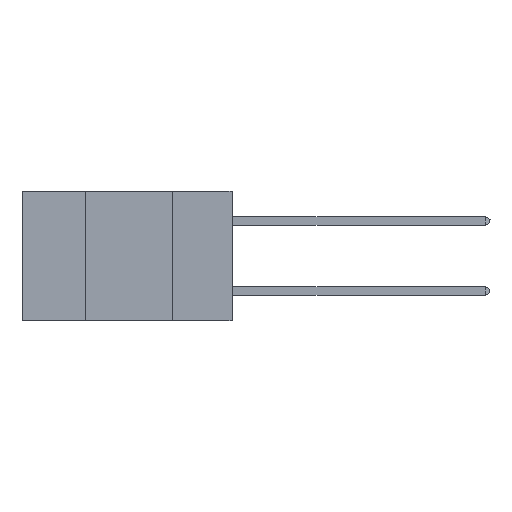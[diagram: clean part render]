
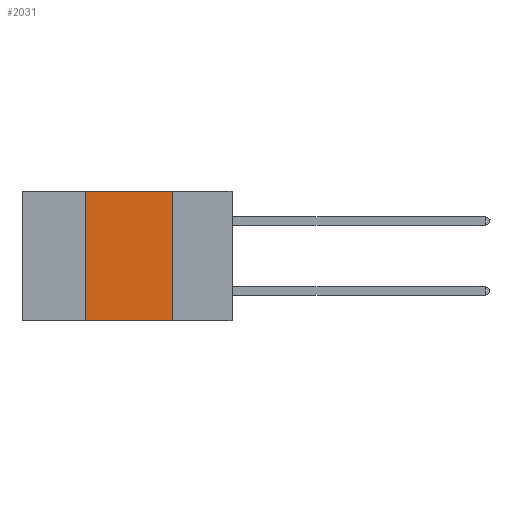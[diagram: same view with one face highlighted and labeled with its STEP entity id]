
A CAD part, left-side view. The second image highlights one B-rep face of the part: STEP entity #2031.
In plain terms, the highlighted planar face has unit normal (-1, 0, 0).
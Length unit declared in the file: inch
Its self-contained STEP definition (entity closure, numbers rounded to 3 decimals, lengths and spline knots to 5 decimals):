
#531 = DIRECTION ( 'NONE',  ( 0., 0., 1. ) ) ;
#580 = EDGE_CURVE ( 'NONE', #26823, #16177, #17739, .T. ) ;
#1506 = DIRECTION ( 'NONE',  ( 0., -1., 0. ) ) ;
#1813 = ORIENTED_EDGE ( 'NONE', *, *, #7496, .F. ) ;
#2031 = ADVANCED_FACE ( 'NONE', ( #20813 ), #12401, .F. ) ;
#2647 = ORIENTED_EDGE ( 'NONE', *, *, #580, .T. ) ;
#3221 = CARTESIAN_POINT ( 'NONE',  ( 0., 0.42, -0.37 ) ) ;
#3333 = CARTESIAN_POINT ( 'NONE',  ( 0., 0.6, 0. ) ) ;
#4228 = CARTESIAN_POINT ( 'NONE',  ( 0., 0.17, 0. ) ) ;
#5326 = VERTEX_POINT ( 'NONE', #15257 ) ;
#6355 = LINE ( 'NONE', #4228, #32613 ) ;
#7496 = EDGE_CURVE ( 'NONE', #26823, #5326, #14928, .T. ) ;
#8200 = CARTESIAN_POINT ( 'NONE',  ( 0., 0.42, 0. ) ) ;
#9907 = VECTOR ( 'NONE', #31317, 39.37008 ) ;
#10989 = CARTESIAN_POINT ( 'NONE',  ( 0., 0.17, -0.37 ) ) ;
#11143 = EDGE_CURVE ( 'NONE', #19741, #16177, #6355, .T. ) ;
#12401 = PLANE ( 'NONE',  #16261 ) ;
#13362 = EDGE_LOOP ( 'NONE', ( #13890, #20681, #1813, #2647 ) ) ;
#13890 = ORIENTED_EDGE ( 'NONE', *, *, #11143, .F. ) ;
#14087 = VECTOR ( 'NONE', #531, 39.37008 ) ;
#14613 = DIRECTION ( 'NONE',  ( 0., 0., -1. ) ) ;
#14928 = LINE ( 'NONE', #8200, #14087 ) ;
#15153 = DIRECTION ( 'NONE',  ( 0., 0., -1. ) ) ;
#15257 = CARTESIAN_POINT ( 'NONE',  ( 0., 0.42, 0. ) ) ;
#16177 = VERTEX_POINT ( 'NONE', #10989 ) ;
#16261 = AXIS2_PLACEMENT_3D ( 'NONE', #27712, #30237, #15153 ) ;
#16936 = VECTOR ( 'NONE', #1506, 39.37008 ) ;
#16974 = CARTESIAN_POINT ( 'NONE',  ( 0., 0.6, -0.37 ) ) ;
#17577 = LINE ( 'NONE', #3333, #9907 ) ;
#17739 = LINE ( 'NONE', #16974, #16936 ) ;
#19741 = VERTEX_POINT ( 'NONE', #26836 ) ;
#20681 = ORIENTED_EDGE ( 'NONE', *, *, #28763, .F. ) ;
#20813 = FACE_OUTER_BOUND ( 'NONE', #13362, .T. ) ;
#26823 = VERTEX_POINT ( 'NONE', #3221 ) ;
#26836 = CARTESIAN_POINT ( 'NONE',  ( 0., 0.17, 0. ) ) ;
#27712 = CARTESIAN_POINT ( 'NONE',  ( 0., 0.6, 0. ) ) ;
#28763 = EDGE_CURVE ( 'NONE', #5326, #19741, #17577, .T. ) ;
#30237 = DIRECTION ( 'NONE',  ( 1., 0., 0. ) ) ;
#31317 = DIRECTION ( 'NONE',  ( 0., -1., 0. ) ) ;
#32613 = VECTOR ( 'NONE', #14613, 39.37008 ) ;
